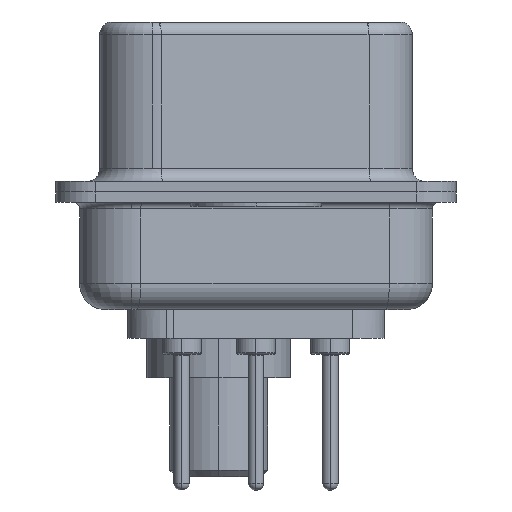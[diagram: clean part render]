
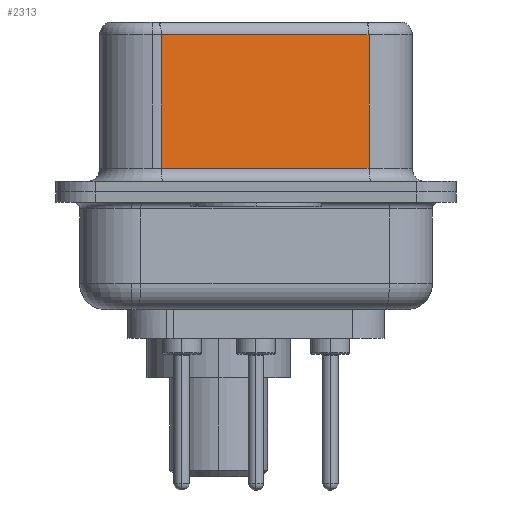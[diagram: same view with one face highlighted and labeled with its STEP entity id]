
A CAD part, left-side view. The second image highlights one B-rep face of the part: STEP entity #2313.
In plain terms, the highlighted planar face has unit normal (-0.985, -0.174, 0).
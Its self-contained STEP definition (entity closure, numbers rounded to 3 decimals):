
#2214 = DIRECTION ( 'NONE',  ( 0.174, -0.985, 0. ) ) ;
#2282 = ORIENTED_EDGE ( 'NONE', *, *, #25856, .T. ) ;
#2301 = EDGE_CURVE ( 'NONE', #14923, #7730, #24134, .T. ) ;
#2313 = ADVANCED_FACE ( 'NONE', ( #2491 ), #11370, .F. ) ;
#2354 = DIRECTION ( 'NONE',  ( 0.985, 0.174, 0. ) ) ;
#2491 = FACE_OUTER_BOUND ( 'NONE', #8454, .T. ) ;
#3372 = VECTOR ( 'NONE', #22306, 1000. ) ;
#3934 = ORIENTED_EDGE ( 'NONE', *, *, #4040, .T. ) ;
#4040 = EDGE_CURVE ( 'NONE', #4938, #7730, #7241, .T. ) ;
#4938 = VERTEX_POINT ( 'NONE', #10226 ) ;
#5616 = CARTESIAN_POINT ( 'NONE',  ( 5.132, -4.322, 6.02 ) ) ;
#5744 = CARTESIAN_POINT ( 'NONE',  ( 5.132, -4.322, 6.52 ) ) ;
#7241 = LINE ( 'NONE', #23537, #17423 ) ;
#7730 = VERTEX_POINT ( 'NONE', #16723 ) ;
#8076 = VECTOR ( 'NONE', #23648, 1000. ) ;
#8454 = EDGE_LOOP ( 'NONE', ( #25361, #16448, #2282, #3934 ) ) ;
#9929 = VECTOR ( 'NONE', #13906, 1000. ) ;
#10226 = CARTESIAN_POINT ( 'NONE',  ( 3.73, 3.628, 0.9 ) ) ;
#10577 = LINE ( 'NONE', #21838, #9929 ) ;
#11370 = PLANE ( 'NONE',  #11682 ) ;
#11682 = AXIS2_PLACEMENT_3D ( 'NONE', #15136, #2354, #16512 ) ;
#13906 = DIRECTION ( 'NONE',  ( -0.174, 0.985, 0. ) ) ;
#14923 = VERTEX_POINT ( 'NONE', #5616 ) ;
#15136 = CARTESIAN_POINT ( 'NONE',  ( 5.132, -4.322, 6.52 ) ) ;
#16448 = ORIENTED_EDGE ( 'NONE', *, *, #25036, .T. ) ;
#16512 = DIRECTION ( 'NONE',  ( -0.174, 0.985, 0. ) ) ;
#16723 = CARTESIAN_POINT ( 'NONE',  ( 5.132, -4.322, 0.9 ) ) ;
#17423 = VECTOR ( 'NONE', #2214, 1000. ) ;
#18403 = CARTESIAN_POINT ( 'NONE',  ( 3.73, 3.628, 6.52 ) ) ;
#18776 = CARTESIAN_POINT ( 'NONE',  ( 3.73, 3.628, 6.02 ) ) ;
#19653 = LINE ( 'NONE', #18403, #3372 ) ;
#20921 = VERTEX_POINT ( 'NONE', #18776 ) ;
#21838 = CARTESIAN_POINT ( 'NONE',  ( 5.132, -4.322, 6.02 ) ) ;
#22306 = DIRECTION ( 'NONE',  ( 0., 0., -1. ) ) ;
#23537 = CARTESIAN_POINT ( 'NONE',  ( 5.132, -4.322, 0.9 ) ) ;
#23648 = DIRECTION ( 'NONE',  ( 0., 0., -1. ) ) ;
#24134 = LINE ( 'NONE', #5744, #8076 ) ;
#25036 = EDGE_CURVE ( 'NONE', #14923, #20921, #10577, .T. ) ;
#25361 = ORIENTED_EDGE ( 'NONE', *, *, #2301, .F. ) ;
#25856 = EDGE_CURVE ( 'NONE', #20921, #4938, #19653, .T. ) ;
